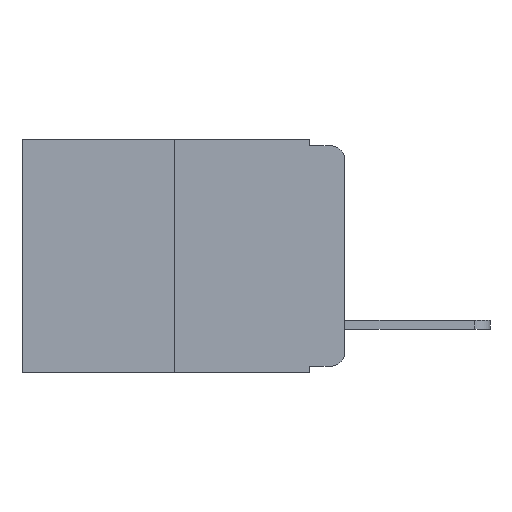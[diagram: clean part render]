
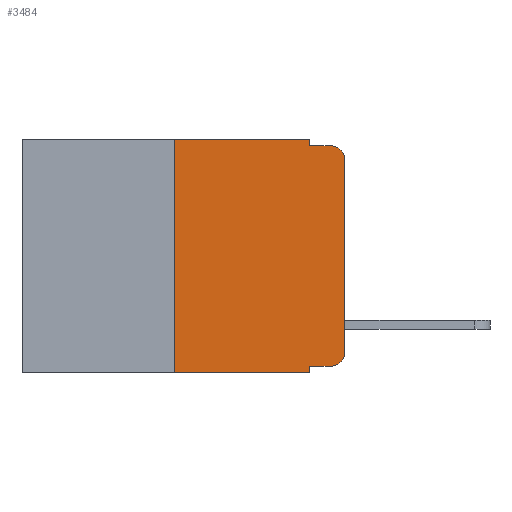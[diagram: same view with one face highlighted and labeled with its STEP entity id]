
A CAD part, left-side view. The second image highlights one B-rep face of the part: STEP entity #3484.
In plain terms, the highlighted planar face has unit normal (-1, 0, 0).
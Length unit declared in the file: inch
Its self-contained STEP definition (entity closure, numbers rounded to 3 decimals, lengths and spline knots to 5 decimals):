
#19 = VECTOR ( 'NONE', #8172, 39.37008 ) ;
#157 = LINE ( 'NONE', #3336, #11377 ) ;
#517 = VERTEX_POINT ( 'NONE', #12347 ) ;
#528 = CARTESIAN_POINT ( 'NONE',  ( 0., 0., -0.03 ) ) ;
#816 = LINE ( 'NONE', #9634, #9507 ) ;
#1063 = VERTEX_POINT ( 'NONE', #10493 ) ;
#1132 = VERTEX_POINT ( 'NONE', #10017 ) ;
#1374 = ORIENTED_EDGE ( 'NONE', *, *, #11459, .F. ) ;
#1625 = EDGE_CURVE ( 'NONE', #1063, #517, #157, .T. ) ;
#1656 = ORIENTED_EDGE ( 'NONE', *, *, #11892, .T. ) ;
#1819 = VERTEX_POINT ( 'NONE', #528 ) ;
#1955 = ORIENTED_EDGE ( 'NONE', *, *, #11531, .F. ) ;
#2219 = CARTESIAN_POINT ( 'NONE',  ( 0., 0.25, -0.343 ) ) ;
#2327 = VERTEX_POINT ( 'NONE', #12977 ) ;
#2355 = ORIENTED_EDGE ( 'NONE', *, *, #7145, .T. ) ;
#2417 = LINE ( 'NONE', #10739, #5195 ) ;
#3020 = DIRECTION ( 'NONE',  ( 0., -1., 0. ) ) ;
#3076 = VERTEX_POINT ( 'NONE', #12063 ) ;
#3298 = ORIENTED_EDGE ( 'NONE', *, *, #11514, .F. ) ;
#3336 = CARTESIAN_POINT ( 'NONE',  ( 0., 0.473, 0. ) ) ;
#3484 = ADVANCED_FACE ( 'NONE', ( #12393 ), #3825, .F. ) ;
#3545 = CARTESIAN_POINT ( 'NONE',  ( 0., 0.02, -0.333 ) ) ;
#3594 = CIRCLE ( 'NONE', #4062, 0.02 ) ;
#3825 = PLANE ( 'NONE',  #9069 ) ;
#3866 = ORIENTED_EDGE ( 'NONE', *, *, #11697, .T. ) ;
#3940 = CARTESIAN_POINT ( 'NONE',  ( 0., 0.473, 0. ) ) ;
#4062 = AXIS2_PLACEMENT_3D ( 'NONE', #11194, #11163, #11153 ) ;
#4093 = ORIENTED_EDGE ( 'NONE', *, *, #1625, .F. ) ;
#4158 = VECTOR ( 'NONE', #9980, 39.37008 ) ;
#4213 = ORIENTED_EDGE ( 'NONE', *, *, #11357, .F. ) ;
#4548 = CARTESIAN_POINT ( 'NONE',  ( 0., 0.02, -0.01 ) ) ;
#4615 = ORIENTED_EDGE ( 'NONE', *, *, #11274, .T. ) ;
#4945 = VERTEX_POINT ( 'NONE', #4548 ) ;
#5018 = DIRECTION ( 'NONE',  ( 0., 0., -1. ) ) ;
#5029 = DIRECTION ( 'NONE',  ( 1., 0., 0. ) ) ;
#5181 = EDGE_LOOP ( 'NONE', ( #1656, #3866, #1955, #3298, #4093, #1374, #2355, #4213, #6836, #4615 ) ) ;
#5195 = VECTOR ( 'NONE', #10642, 39.37008 ) ;
#5458 = VERTEX_POINT ( 'NONE', #2219 ) ;
#5522 = VECTOR ( 'NONE', #10864, 39.37008 ) ;
#6011 = VERTEX_POINT ( 'NONE', #3545 ) ;
#6380 = DIRECTION ( 'NONE',  ( 0., 0., 1. ) ) ;
#6547 = CARTESIAN_POINT ( 'NONE',  ( 0., 0., 0. ) ) ;
#6756 = VERTEX_POINT ( 'NONE', #13224 ) ;
#6836 = ORIENTED_EDGE ( 'NONE', *, *, #11308, .T. ) ;
#7143 = LINE ( 'NONE', #10063, #4158 ) ;
#7145 = EDGE_CURVE ( 'NONE', #5458, #3076, #8853, .T. ) ;
#7967 = CIRCLE ( 'NONE', #9743, 0.02 ) ;
#8131 = DIRECTION ( 'NONE',  ( 0., 0., -1. ) ) ;
#8172 = DIRECTION ( 'NONE',  ( 0., -1., 0. ) ) ;
#8174 = CARTESIAN_POINT ( 'NONE',  ( 0., 0.473, -0.343 ) ) ;
#8213 = DIRECTION ( 'NONE',  ( -1., 0., 0. ) ) ;
#8280 = CARTESIAN_POINT ( 'NONE',  ( 0., 0.02, -0.03 ) ) ;
#8419 = VECTOR ( 'NONE', #6380, 39.37008 ) ;
#8853 = LINE ( 'NONE', #8174, #19 ) ;
#9069 = AXIS2_PLACEMENT_3D ( 'NONE', #3940, #5029, #5018 ) ;
#9412 = DIRECTION ( 'NONE',  ( 0., -1., 0. ) ) ;
#9439 = CARTESIAN_POINT ( 'NONE',  ( 0., 0.051, -0.01 ) ) ;
#9507 = VECTOR ( 'NONE', #9511, 39.37008 ) ;
#9511 = DIRECTION ( 'NONE',  ( 0., 0., -1. ) ) ;
#9634 = CARTESIAN_POINT ( 'NONE',  ( 0., 0.051, 0. ) ) ;
#9743 = AXIS2_PLACEMENT_3D ( 'NONE', #8280, #8213, #8131 ) ;
#9980 = DIRECTION ( 'NONE',  ( 0., 0., 1. ) ) ;
#10017 = CARTESIAN_POINT ( 'NONE',  ( 0., 0.051, -0.01 ) ) ;
#10063 = CARTESIAN_POINT ( 'NONE',  ( 0., 0.25, 0. ) ) ;
#10493 = CARTESIAN_POINT ( 'NONE',  ( 0., 0.25, 0. ) ) ;
#10642 = DIRECTION ( 'NONE',  ( 0., 0., -1. ) ) ;
#10739 = CARTESIAN_POINT ( 'NONE',  ( 0., 0.051, 0. ) ) ;
#10864 = DIRECTION ( 'NONE',  ( 0., -1., 0. ) ) ;
#10880 = CARTESIAN_POINT ( 'NONE',  ( 0., 0.051, -0.333 ) ) ;
#10909 = LINE ( 'NONE', #6547, #8419 ) ;
#11153 = DIRECTION ( 'NONE',  ( 0., 0., -1. ) ) ;
#11163 = DIRECTION ( 'NONE',  ( -1., 0., 0. ) ) ;
#11194 = CARTESIAN_POINT ( 'NONE',  ( 0., 0.02, -0.313 ) ) ;
#11274 = EDGE_CURVE ( 'NONE', #6011, #2327, #3594, .T. ) ;
#11308 = EDGE_CURVE ( 'NONE', #6756, #6011, #13200, .T. ) ;
#11330 = VECTOR ( 'NONE', #9412, 39.37008 ) ;
#11357 = EDGE_CURVE ( 'NONE', #6756, #3076, #2417, .T. ) ;
#11377 = VECTOR ( 'NONE', #3020, 39.37008 ) ;
#11459 = EDGE_CURVE ( 'NONE', #5458, #1063, #7143, .T. ) ;
#11514 = EDGE_CURVE ( 'NONE', #517, #1132, #816, .T. ) ;
#11531 = EDGE_CURVE ( 'NONE', #1132, #4945, #11608, .T. ) ;
#11608 = LINE ( 'NONE', #9439, #11330 ) ;
#11697 = EDGE_CURVE ( 'NONE', #1819, #4945, #7967, .T. ) ;
#11892 = EDGE_CURVE ( 'NONE', #2327, #1819, #10909, .T. ) ;
#12063 = CARTESIAN_POINT ( 'NONE',  ( 0., 0.051, -0.343 ) ) ;
#12347 = CARTESIAN_POINT ( 'NONE',  ( 0., 0.051, 0. ) ) ;
#12393 = FACE_OUTER_BOUND ( 'NONE', #5181, .T. ) ;
#12977 = CARTESIAN_POINT ( 'NONE',  ( 0., 0., -0.313 ) ) ;
#13200 = LINE ( 'NONE', #10880, #5522 ) ;
#13224 = CARTESIAN_POINT ( 'NONE',  ( 0., 0.051, -0.333 ) ) ;
